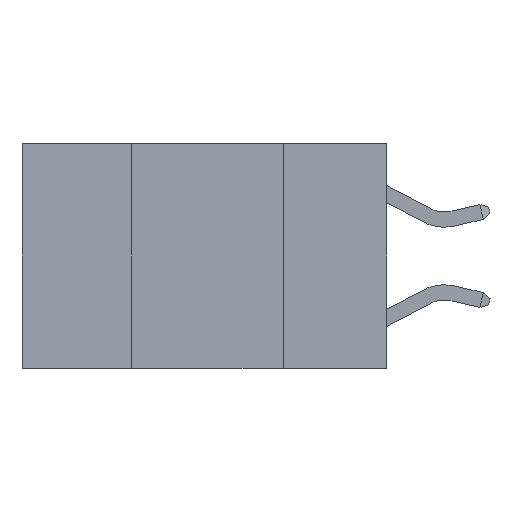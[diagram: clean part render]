
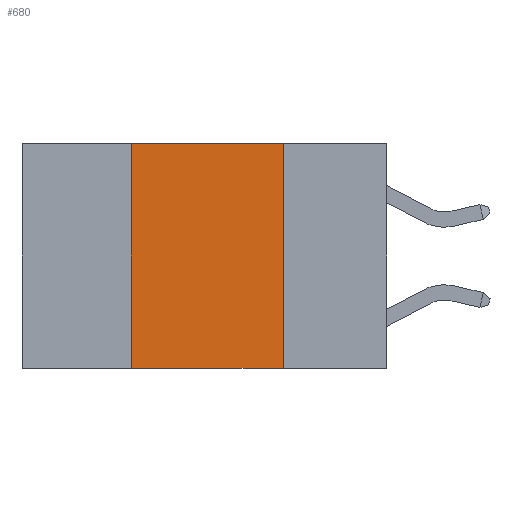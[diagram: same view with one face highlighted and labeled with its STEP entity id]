
A CAD part, left-side view. The second image highlights one B-rep face of the part: STEP entity #680.
In plain terms, the highlighted planar face has unit normal (-1, 0, 0).
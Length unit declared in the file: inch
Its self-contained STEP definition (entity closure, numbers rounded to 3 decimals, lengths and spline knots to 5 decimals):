
#125 = LINE ( 'NONE', #6515, #11587 ) ;
#157 = DIRECTION ( 'NONE',  ( 0., 0., 1. ) ) ;
#597 = CARTESIAN_POINT ( 'NONE',  ( 0., 0.17, 0. ) ) ;
#680 = ADVANCED_FACE ( 'NONE', ( #11196 ), #9428, .F. ) ;
#927 = DIRECTION ( 'NONE',  ( 0., -1., 0. ) ) ;
#1012 = EDGE_CURVE ( 'NONE', #7834, #3905, #4878, .T. ) ;
#1164 = CARTESIAN_POINT ( 'NONE',  ( 0., 0.17, 0. ) ) ;
#1213 = ORIENTED_EDGE ( 'NONE', *, *, #10813, .F. ) ;
#1312 = CARTESIAN_POINT ( 'NONE',  ( 0., 0.17, -0.37 ) ) ;
#2097 = DIRECTION ( 'NONE',  ( 0., 0., -1. ) ) ;
#3632 = ORIENTED_EDGE ( 'NONE', *, *, #1012, .F. ) ;
#3697 = DIRECTION ( 'NONE',  ( 0., -1., 0. ) ) ;
#3772 = DIRECTION ( 'NONE',  ( 1., 0., 0. ) ) ;
#3905 = VERTEX_POINT ( 'NONE', #597 ) ;
#4629 = CARTESIAN_POINT ( 'NONE',  ( 0., 0.6, 0. ) ) ;
#4878 = LINE ( 'NONE', #4629, #9389 ) ;
#5649 = CARTESIAN_POINT ( 'NONE',  ( 0., 0.42, 0. ) ) ;
#6011 = VERTEX_POINT ( 'NONE', #1312 ) ;
#6398 = LINE ( 'NONE', #1164, #8529 ) ;
#6515 = CARTESIAN_POINT ( 'NONE',  ( 0., 0.42, 0. ) ) ;
#6856 = EDGE_LOOP ( 'NONE', ( #1213, #3632, #6868, #9272 ) ) ;
#6868 = ORIENTED_EDGE ( 'NONE', *, *, #11487, .F. ) ;
#7221 = VERTEX_POINT ( 'NONE', #10315 ) ;
#7247 = CARTESIAN_POINT ( 'NONE',  ( 0., 0.6, -0.37 ) ) ;
#7828 = CARTESIAN_POINT ( 'NONE',  ( 0., 0.6, 0. ) ) ;
#7834 = VERTEX_POINT ( 'NONE', #5649 ) ;
#8051 = AXIS2_PLACEMENT_3D ( 'NONE', #7828, #3772, #8326 ) ;
#8326 = DIRECTION ( 'NONE',  ( 0., 0., -1. ) ) ;
#8529 = VECTOR ( 'NONE', #2097, 39.37008 ) ;
#8861 = EDGE_CURVE ( 'NONE', #7221, #6011, #9286, .T. ) ;
#9272 = ORIENTED_EDGE ( 'NONE', *, *, #8861, .T. ) ;
#9286 = LINE ( 'NONE', #7247, #11377 ) ;
#9389 = VECTOR ( 'NONE', #3697, 39.37008 ) ;
#9428 = PLANE ( 'NONE',  #8051 ) ;
#10315 = CARTESIAN_POINT ( 'NONE',  ( 0., 0.42, -0.37 ) ) ;
#10813 = EDGE_CURVE ( 'NONE', #3905, #6011, #6398, .T. ) ;
#11196 = FACE_OUTER_BOUND ( 'NONE', #6856, .T. ) ;
#11377 = VECTOR ( 'NONE', #927, 39.37008 ) ;
#11487 = EDGE_CURVE ( 'NONE', #7221, #7834, #125, .T. ) ;
#11587 = VECTOR ( 'NONE', #157, 39.37008 ) ;
